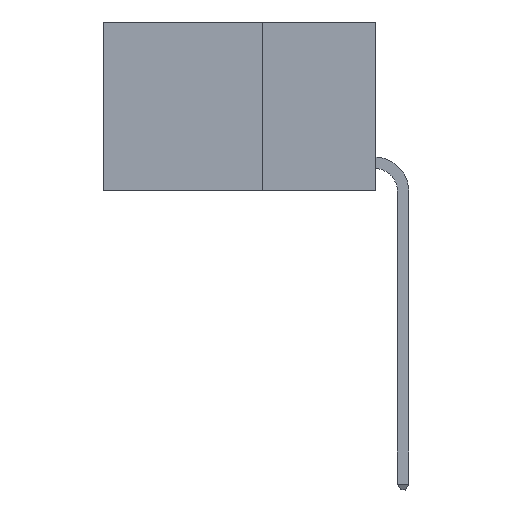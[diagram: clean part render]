
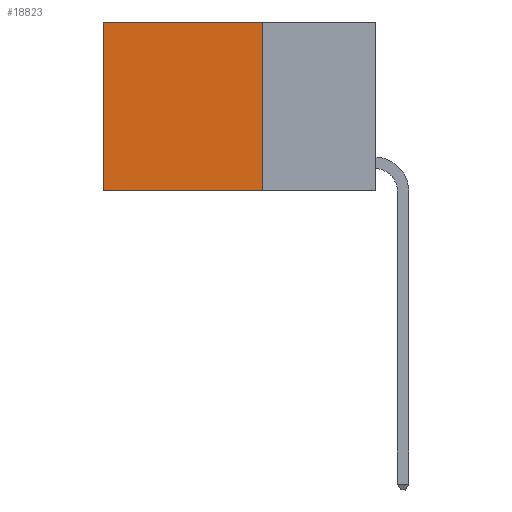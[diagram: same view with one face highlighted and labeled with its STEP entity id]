
A CAD part, left-side view. The second image highlights one B-rep face of the part: STEP entity #18823.
In plain terms, the highlighted planar face has unit normal (-1, 0, 0).
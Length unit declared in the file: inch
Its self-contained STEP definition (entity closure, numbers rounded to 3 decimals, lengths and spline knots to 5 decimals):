
#77 = LINE ( 'NONE', #25945, #5479 ) ;
#379 = CARTESIAN_POINT ( 'NONE',  ( 0.2625, 0.25, 0. ) ) ;
#2302 = DIRECTION ( 'NONE',  ( 0., 0., -1. ) ) ;
#3501 = CARTESIAN_POINT ( 'NONE',  ( 0.2625, 0.6, 0. ) ) ;
#4024 = EDGE_LOOP ( 'NONE', ( #16442, #26944, #15157, #21039 ) ) ;
#5479 = VECTOR ( 'NONE', #28188, 39.37008 ) ;
#6008 = AXIS2_PLACEMENT_3D ( 'NONE', #29304, #16053, #2302 ) ;
#6046 = CARTESIAN_POINT ( 'NONE',  ( 0.2625, 0.25, -0.37 ) ) ;
#9533 = VERTEX_POINT ( 'NONE', #6046 ) ;
#10001 = LINE ( 'NONE', #3501, #15415 ) ;
#12167 = DIRECTION ( 'NONE',  ( 0., 0., -1. ) ) ;
#13251 = VECTOR ( 'NONE', #12167, 39.37008 ) ;
#15157 = ORIENTED_EDGE ( 'NONE', *, *, #21268, .F. ) ;
#15415 = VECTOR ( 'NONE', #19477, 39.37008 ) ;
#15540 = CARTESIAN_POINT ( 'NONE',  ( 0.2625, 0.6, 0. ) ) ;
#15553 = CARTESIAN_POINT ( 'NONE',  ( 0.2625, 0.6, -0.37 ) ) ;
#15674 = VERTEX_POINT ( 'NONE', #379 ) ;
#16053 = DIRECTION ( 'NONE',  ( 1., 0., 0. ) ) ;
#16060 = VERTEX_POINT ( 'NONE', #15540 ) ;
#16442 = ORIENTED_EDGE ( 'NONE', *, *, #20529, .T. ) ;
#17177 = VECTOR ( 'NONE', #20759, 39.37008 ) ;
#18823 = ADVANCED_FACE ( 'NONE', ( #25274 ), #20430, .F. ) ;
#19267 = LINE ( 'NONE', #21174, #13251 ) ;
#19477 = DIRECTION ( 'NONE',  ( 0., 0., -1. ) ) ;
#20235 = EDGE_CURVE ( 'NONE', #9533, #24359, #23786, .T. ) ;
#20430 = PLANE ( 'NONE',  #6008 ) ;
#20529 = EDGE_CURVE ( 'NONE', #16060, #24359, #10001, .T. ) ;
#20759 = DIRECTION ( 'NONE',  ( 0., 1., 0. ) ) ;
#21039 = ORIENTED_EDGE ( 'NONE', *, *, #27659, .T. ) ;
#21174 = CARTESIAN_POINT ( 'NONE',  ( 0.2625, 0.25, 0. ) ) ;
#21268 = EDGE_CURVE ( 'NONE', #15674, #9533, #19267, .T. ) ;
#23786 = LINE ( 'NONE', #27370, #17177 ) ;
#24359 = VERTEX_POINT ( 'NONE', #15553 ) ;
#25274 = FACE_OUTER_BOUND ( 'NONE', #4024, .T. ) ;
#25945 = CARTESIAN_POINT ( 'NONE',  ( 0.2625, 0.25, 0. ) ) ;
#26944 = ORIENTED_EDGE ( 'NONE', *, *, #20235, .F. ) ;
#27370 = CARTESIAN_POINT ( 'NONE',  ( 0.2625, 0.25, -0.37 ) ) ;
#27659 = EDGE_CURVE ( 'NONE', #15674, #16060, #77, .T. ) ;
#28188 = DIRECTION ( 'NONE',  ( 0., 1., 0. ) ) ;
#29304 = CARTESIAN_POINT ( 'NONE',  ( 0.2625, 0.25, 0. ) ) ;
